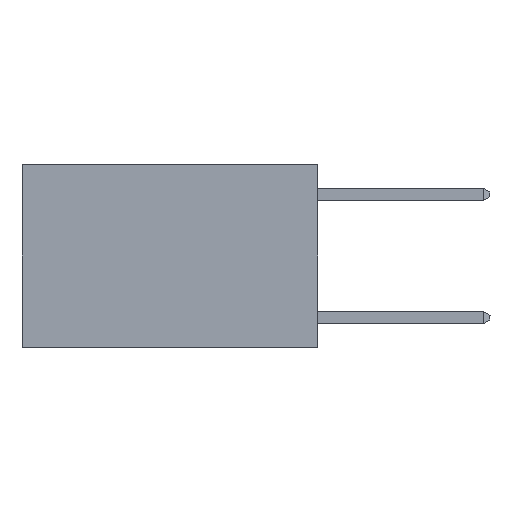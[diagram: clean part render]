
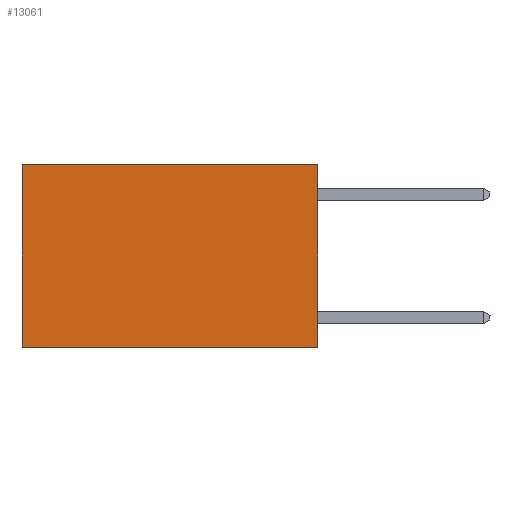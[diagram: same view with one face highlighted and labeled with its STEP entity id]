
A CAD part, left-side view. The second image highlights one B-rep face of the part: STEP entity #13061.
In plain terms, the highlighted planar face has unit normal (-1, 0, 0).
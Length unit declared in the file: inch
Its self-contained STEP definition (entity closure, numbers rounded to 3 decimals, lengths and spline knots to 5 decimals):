
#354 = DIRECTION ( 'NONE',  ( 0., 1., 0. ) ) ;
#1906 = VECTOR ( 'NONE', #23022, 39.37008 ) ;
#2556 = CARTESIAN_POINT ( 'NONE',  ( 0.2625, 0.6, 0. ) ) ;
#2721 = VECTOR ( 'NONE', #22490, 39.37008 ) ;
#3366 = VERTEX_POINT ( 'NONE', #10513 ) ;
#7025 = DIRECTION ( 'NONE',  ( 0., 0., -1. ) ) ;
#7188 = CARTESIAN_POINT ( 'NONE',  ( 0.2625, 0., -0.37 ) ) ;
#7419 = EDGE_CURVE ( 'NONE', #20469, #11672, #10886, .T. ) ;
#7745 = PLANE ( 'NONE',  #14222 ) ;
#7855 = DIRECTION ( 'NONE',  ( 0., 0., -1. ) ) ;
#7919 = EDGE_CURVE ( 'NONE', #11672, #13637, #25402, .T. ) ;
#9745 = EDGE_LOOP ( 'NONE', ( #17229, #17687, #17855, #18198 ) ) ;
#10513 = CARTESIAN_POINT ( 'NONE',  ( 0.2625, 0., -0.37 ) ) ;
#10886 = LINE ( 'NONE', #26534, #17435 ) ;
#11672 = VERTEX_POINT ( 'NONE', #20396 ) ;
#12416 = CARTESIAN_POINT ( 'NONE',  ( 0.2625, 0.6, -0.37 ) ) ;
#13061 = ADVANCED_FACE ( 'NONE', ( #18380 ), #7745, .F. ) ;
#13637 = VERTEX_POINT ( 'NONE', #12416 ) ;
#13693 = LINE ( 'NONE', #20846, #1906 ) ;
#14210 = CARTESIAN_POINT ( 'NONE',  ( 0.2625, 0., 0. ) ) ;
#14222 = AXIS2_PLACEMENT_3D ( 'NONE', #14210, #20931, #7855 ) ;
#17229 = ORIENTED_EDGE ( 'NONE', *, *, #7919, .T. ) ;
#17435 = VECTOR ( 'NONE', #354, 39.37008 ) ;
#17687 = ORIENTED_EDGE ( 'NONE', *, *, #21575, .F. ) ;
#17855 = ORIENTED_EDGE ( 'NONE', *, *, #27768, .F. ) ;
#18198 = ORIENTED_EDGE ( 'NONE', *, *, #7419, .T. ) ;
#18380 = FACE_OUTER_BOUND ( 'NONE', #9745, .T. ) ;
#19634 = LINE ( 'NONE', #7188, #2721 ) ;
#19726 = VECTOR ( 'NONE', #7025, 39.37008 ) ;
#20396 = CARTESIAN_POINT ( 'NONE',  ( 0.2625, 0.6, 0. ) ) ;
#20469 = VERTEX_POINT ( 'NONE', #25325 ) ;
#20846 = CARTESIAN_POINT ( 'NONE',  ( 0.2625, 0., 0. ) ) ;
#20931 = DIRECTION ( 'NONE',  ( 1., 0., 0. ) ) ;
#21575 = EDGE_CURVE ( 'NONE', #3366, #13637, #19634, .T. ) ;
#22490 = DIRECTION ( 'NONE',  ( 0., 1., 0. ) ) ;
#23022 = DIRECTION ( 'NONE',  ( 0., 0., -1. ) ) ;
#25325 = CARTESIAN_POINT ( 'NONE',  ( 0.2625, 0., 0. ) ) ;
#25402 = LINE ( 'NONE', #2556, #19726 ) ;
#26534 = CARTESIAN_POINT ( 'NONE',  ( 0.2625, 0., 0. ) ) ;
#27768 = EDGE_CURVE ( 'NONE', #20469, #3366, #13693, .T. ) ;
